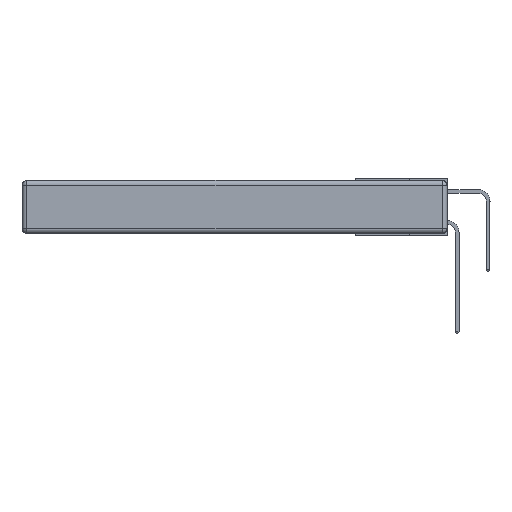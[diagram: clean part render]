
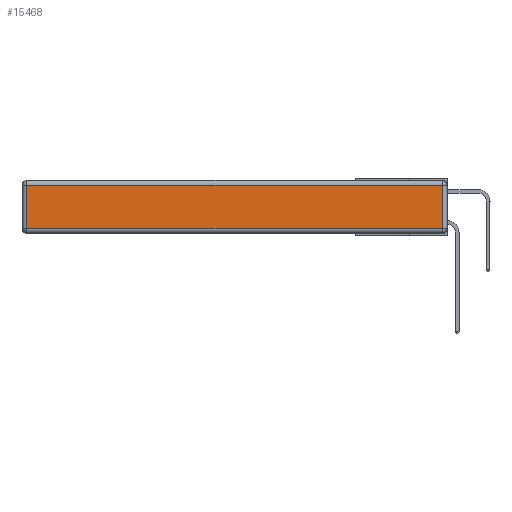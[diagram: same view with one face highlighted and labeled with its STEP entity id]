
A CAD part, left-side view. The second image highlights one B-rep face of the part: STEP entity #15468.
In plain terms, the highlighted planar face has unit normal (-1, 0, 0).
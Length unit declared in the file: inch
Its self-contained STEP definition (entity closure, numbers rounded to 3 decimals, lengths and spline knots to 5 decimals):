
#662 = ORIENTED_EDGE ( 'NONE', *, *, #26784, .T. ) ;
#1050 = ORIENTED_EDGE ( 'NONE', *, *, #21262, .T. ) ;
#1192 = LINE ( 'NONE', #20058, #16043 ) ;
#1868 = AXIS2_PLACEMENT_3D ( 'NONE', #23578, #7120, #5062 ) ;
#3275 = FACE_OUTER_BOUND ( 'NONE', #5257, .T. ) ;
#5062 = DIRECTION ( 'NONE',  ( 0., 0., 1. ) ) ;
#5257 = EDGE_LOOP ( 'NONE', ( #1050, #17396, #29348, #662 ) ) ;
#7120 = DIRECTION ( 'NONE',  ( -1., 0., 0. ) ) ;
#9481 = PLANE ( 'NONE',  #1868 ) ;
#12292 = CARTESIAN_POINT ( 'NONE',  ( 0., 0.03, -0.343 ) ) ;
#12769 = VERTEX_POINT ( 'NONE', #22697 ) ;
#13348 = DIRECTION ( 'NONE',  ( 0., 1., 0. ) ) ;
#14136 = CARTESIAN_POINT ( 'NONE',  ( 0., 2.75, -0.03 ) ) ;
#15468 = ADVANCED_FACE ( 'NONE', ( #3275 ), #9481, .T. ) ;
#16043 = VECTOR ( 'NONE', #29563, 39.37008 ) ;
#17396 = ORIENTED_EDGE ( 'NONE', *, *, #17507, .T. ) ;
#17507 = EDGE_CURVE ( 'NONE', #21230, #12769, #29553, .T. ) ;
#17522 = LINE ( 'NONE', #28059, #26386 ) ;
#18706 = DIRECTION ( 'NONE',  ( 0., 0., -1. ) ) ;
#18815 = VECTOR ( 'NONE', #28643, 39.37008 ) ;
#20058 = CARTESIAN_POINT ( 'NONE',  ( 0., 0., -0.313 ) ) ;
#20593 = CARTESIAN_POINT ( 'NONE',  ( 0., 2.72, -0.313 ) ) ;
#21230 = VERTEX_POINT ( 'NONE', #27058 ) ;
#21262 = EDGE_CURVE ( 'NONE', #27905, #21230, #1192, .T. ) ;
#22697 = CARTESIAN_POINT ( 'NONE',  ( 0., 0.03, -0.03 ) ) ;
#23578 = CARTESIAN_POINT ( 'NONE',  ( 0., 0., -0.343 ) ) ;
#23895 = VECTOR ( 'NONE', #13348, 39.37008 ) ;
#24224 = LINE ( 'NONE', #14136, #23895 ) ;
#25198 = EDGE_CURVE ( 'NONE', #12769, #29482, #24224, .T. ) ;
#26386 = VECTOR ( 'NONE', #18706, 39.37008 ) ;
#26618 = CARTESIAN_POINT ( 'NONE',  ( 0., 2.72, -0.03 ) ) ;
#26784 = EDGE_CURVE ( 'NONE', #29482, #27905, #17522, .T. ) ;
#27058 = CARTESIAN_POINT ( 'NONE',  ( 0., 0.03, -0.313 ) ) ;
#27905 = VERTEX_POINT ( 'NONE', #20593 ) ;
#28059 = CARTESIAN_POINT ( 'NONE',  ( 0., 2.72, -0.343 ) ) ;
#28643 = DIRECTION ( 'NONE',  ( 0., 0., 1. ) ) ;
#29348 = ORIENTED_EDGE ( 'NONE', *, *, #25198, .T. ) ;
#29482 = VERTEX_POINT ( 'NONE', #26618 ) ;
#29553 = LINE ( 'NONE', #12292, #18815 ) ;
#29563 = DIRECTION ( 'NONE',  ( 0., -1., 0. ) ) ;
